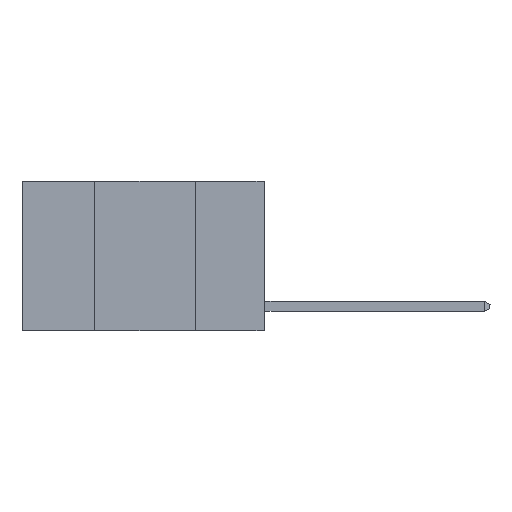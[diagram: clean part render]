
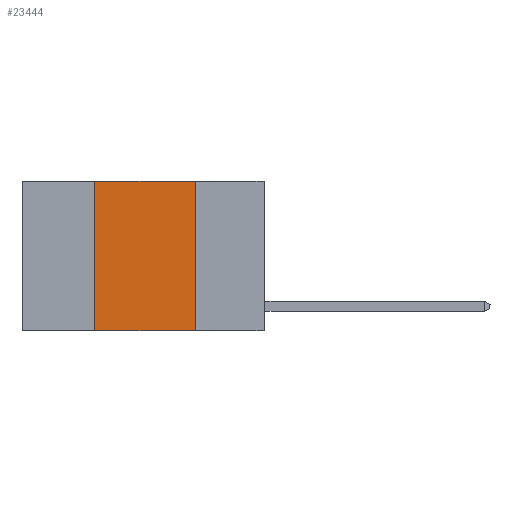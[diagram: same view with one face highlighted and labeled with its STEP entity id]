
A CAD part, left-side view. The second image highlights one B-rep face of the part: STEP entity #23444.
In plain terms, the highlighted planar face has unit normal (-1, 0, 0).
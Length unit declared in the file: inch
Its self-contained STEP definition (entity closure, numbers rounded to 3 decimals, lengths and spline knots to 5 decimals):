
#638 = ORIENTED_EDGE ( 'NONE', *, *, #7953, .F. ) ;
#1119 = DIRECTION ( 'NONE',  ( 1., 0., 0. ) ) ;
#1901 = CARTESIAN_POINT ( 'NONE',  ( 0., 0.42, 0. ) ) ;
#3162 = DIRECTION ( 'NONE',  ( 0., 0., 1. ) ) ;
#3237 = VECTOR ( 'NONE', #13838, 39.37008 ) ;
#4237 = CARTESIAN_POINT ( 'NONE',  ( 0., 0.6, 0. ) ) ;
#4295 = ORIENTED_EDGE ( 'NONE', *, *, #17244, .F. ) ;
#5543 = ORIENTED_EDGE ( 'NONE', *, *, #9688, .T. ) ;
#7668 = LINE ( 'NONE', #19925, #17660 ) ;
#7953 = EDGE_CURVE ( 'NONE', #20998, #21944, #7668, .T. ) ;
#8264 = VERTEX_POINT ( 'NONE', #1901 ) ;
#8453 = CARTESIAN_POINT ( 'NONE',  ( 0., 0.6, -0.37 ) ) ;
#8777 = DIRECTION ( 'NONE',  ( 0., 0., -1. ) ) ;
#9688 = EDGE_CURVE ( 'NONE', #12398, #21944, #13526, .T. ) ;
#10724 = CARTESIAN_POINT ( 'NONE',  ( 0., 0.6, 0. ) ) ;
#12398 = VERTEX_POINT ( 'NONE', #17820 ) ;
#12533 = AXIS2_PLACEMENT_3D ( 'NONE', #10724, #1119, #14507 ) ;
#13526 = LINE ( 'NONE', #8453, #18442 ) ;
#13838 = DIRECTION ( 'NONE',  ( 0., -1., 0. ) ) ;
#13988 = CARTESIAN_POINT ( 'NONE',  ( 0., 0.17, 0. ) ) ;
#14507 = DIRECTION ( 'NONE',  ( 0., 0., -1. ) ) ;
#17099 = FACE_OUTER_BOUND ( 'NONE', #23323, .T. ) ;
#17244 = EDGE_CURVE ( 'NONE', #12398, #8264, #19048, .T. ) ;
#17660 = VECTOR ( 'NONE', #8777, 39.37008 ) ;
#17820 = CARTESIAN_POINT ( 'NONE',  ( 0., 0.42, -0.37 ) ) ;
#18350 = LINE ( 'NONE', #4237, #3237 ) ;
#18442 = VECTOR ( 'NONE', #21433, 39.37008 ) ;
#18772 = ORIENTED_EDGE ( 'NONE', *, *, #20914, .F. ) ;
#19048 = LINE ( 'NONE', #23648, #23234 ) ;
#19925 = CARTESIAN_POINT ( 'NONE',  ( 0., 0.17, 0. ) ) ;
#20914 = EDGE_CURVE ( 'NONE', #8264, #20998, #18350, .T. ) ;
#20998 = VERTEX_POINT ( 'NONE', #13988 ) ;
#21433 = DIRECTION ( 'NONE',  ( 0., -1., 0. ) ) ;
#21944 = VERTEX_POINT ( 'NONE', #24041 ) ;
#23234 = VECTOR ( 'NONE', #3162, 39.37008 ) ;
#23323 = EDGE_LOOP ( 'NONE', ( #638, #18772, #4295, #5543 ) ) ;
#23444 = ADVANCED_FACE ( 'NONE', ( #17099 ), #23570, .F. ) ;
#23570 = PLANE ( 'NONE',  #12533 ) ;
#23648 = CARTESIAN_POINT ( 'NONE',  ( 0., 0.42, 0. ) ) ;
#24041 = CARTESIAN_POINT ( 'NONE',  ( 0., 0.17, -0.37 ) ) ;
